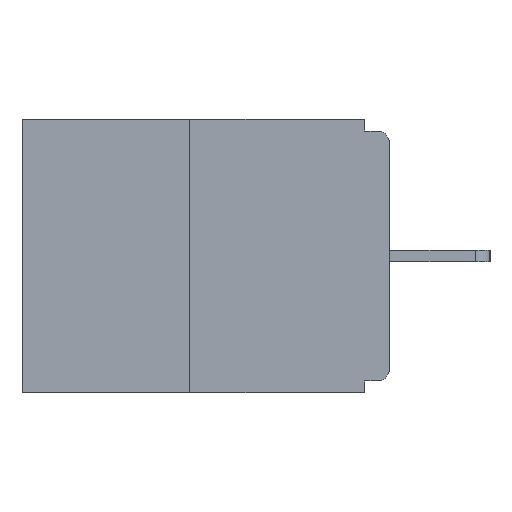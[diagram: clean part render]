
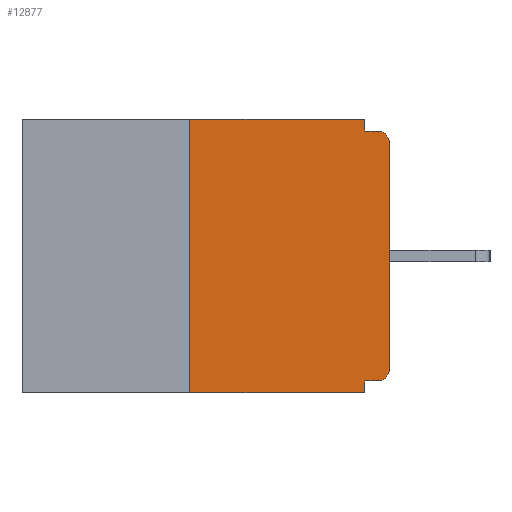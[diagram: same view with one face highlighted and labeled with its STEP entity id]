
A CAD part, left-side view. The second image highlights one B-rep face of the part: STEP entity #12877.
In plain terms, the highlighted planar face has unit normal (-1, 0, 0).
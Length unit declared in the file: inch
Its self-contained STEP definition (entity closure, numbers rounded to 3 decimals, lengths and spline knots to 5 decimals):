
#268 = EDGE_CURVE ( 'NONE', #17005, #15271, #13003, .T. ) ;
#376 = EDGE_CURVE ( 'NONE', #23818, #16217, #7460, .T. ) ;
#537 = LINE ( 'NONE', #25240, #22893 ) ;
#1853 = DIRECTION ( 'NONE',  ( 0., 0., 1. ) ) ;
#2669 = VECTOR ( 'NONE', #3980, 39.37008 ) ;
#2848 = DIRECTION ( 'NONE',  ( 0., 0., -1. ) ) ;
#2906 = VERTEX_POINT ( 'NONE', #8200 ) ;
#3591 = CIRCLE ( 'NONE', #9228, 0.015 ) ;
#3841 = CARTESIAN_POINT ( 'NONE',  ( 0., 0.015, -0.328 ) ) ;
#3980 = DIRECTION ( 'NONE',  ( 0., 0., -1. ) ) ;
#4024 = CARTESIAN_POINT ( 'NONE',  ( 0., 0., 0. ) ) ;
#4127 = AXIS2_PLACEMENT_3D ( 'NONE', #17732, #13574, #5185 ) ;
#4863 = CARTESIAN_POINT ( 'NONE',  ( 0., 0.015, -0.015 ) ) ;
#5080 = FACE_OUTER_BOUND ( 'NONE', #23691, .T. ) ;
#5173 = VECTOR ( 'NONE', #19610, 39.37008 ) ;
#5185 = DIRECTION ( 'NONE',  ( 0., 0., -1. ) ) ;
#5927 = VECTOR ( 'NONE', #1853, 39.37008 ) ;
#6051 = ORIENTED_EDGE ( 'NONE', *, *, #376, .F. ) ;
#6130 = EDGE_CURVE ( 'NONE', #23818, #2906, #10619, .T. ) ;
#6712 = VECTOR ( 'NONE', #8015, 39.37008 ) ;
#7460 = LINE ( 'NONE', #13792, #6712 ) ;
#8015 = DIRECTION ( 'NONE',  ( 0., 1., 0. ) ) ;
#8200 = CARTESIAN_POINT ( 'NONE',  ( 0., 0., -0.313 ) ) ;
#9228 = AXIS2_PLACEMENT_3D ( 'NONE', #24855, #12466, #20682 ) ;
#9291 = EDGE_CURVE ( 'NONE', #2906, #23727, #24266, .T. ) ;
#9389 = CARTESIAN_POINT ( 'NONE',  ( 0., 0.25, 0. ) ) ;
#9894 = CARTESIAN_POINT ( 'NONE',  ( 0., 0.031, 0. ) ) ;
#9942 = ORIENTED_EDGE ( 'NONE', *, *, #14783, .F. ) ;
#10184 = VECTOR ( 'NONE', #25661, 39.37008 ) ;
#10459 = DIRECTION ( 'NONE',  ( 0., -1., 0. ) ) ;
#10619 = CIRCLE ( 'NONE', #4127, 0.015 ) ;
#11185 = DIRECTION ( 'NONE',  ( 0., 0., -1. ) ) ;
#11404 = LINE ( 'NONE', #9389, #5173 ) ;
#11454 = DIRECTION ( 'NONE',  ( 1., 0., 0. ) ) ;
#11769 = VERTEX_POINT ( 'NONE', #14636 ) ;
#12466 = DIRECTION ( 'NONE',  ( -1., 0., 0. ) ) ;
#12542 = ORIENTED_EDGE ( 'NONE', *, *, #268, .F. ) ;
#12877 = ADVANCED_FACE ( 'NONE', ( #5080 ), #23568, .F. ) ;
#12882 = CARTESIAN_POINT ( 'NONE',  ( 0., 0.031, -0.328 ) ) ;
#13003 = LINE ( 'NONE', #17577, #10184 ) ;
#13457 = CARTESIAN_POINT ( 'NONE',  ( 0., 0.46, 0. ) ) ;
#13574 = DIRECTION ( 'NONE',  ( -1., 0., 0. ) ) ;
#13792 = CARTESIAN_POINT ( 'NONE',  ( 0., 0., -0.328 ) ) ;
#14130 = EDGE_CURVE ( 'NONE', #24259, #18812, #537, .T. ) ;
#14636 = CARTESIAN_POINT ( 'NONE',  ( 0., 0.031, -0.343 ) ) ;
#14783 = EDGE_CURVE ( 'NONE', #18812, #17005, #16258, .T. ) ;
#15094 = ORIENTED_EDGE ( 'NONE', *, *, #17762, .T. ) ;
#15271 = VERTEX_POINT ( 'NONE', #4863 ) ;
#15834 = ORIENTED_EDGE ( 'NONE', *, *, #25152, .T. ) ;
#16217 = VERTEX_POINT ( 'NONE', #12882 ) ;
#16241 = EDGE_CURVE ( 'NONE', #16217, #11769, #25123, .T. ) ;
#16258 = LINE ( 'NONE', #24494, #2669 ) ;
#16905 = CARTESIAN_POINT ( 'NONE',  ( 0., 0.25, -0.343 ) ) ;
#17005 = VERTEX_POINT ( 'NONE', #21390 ) ;
#17158 = CARTESIAN_POINT ( 'NONE',  ( 0., 0.031, -0.343 ) ) ;
#17433 = ORIENTED_EDGE ( 'NONE', *, *, #9291, .T. ) ;
#17577 = CARTESIAN_POINT ( 'NONE',  ( 0., 0., -0.015 ) ) ;
#17586 = ORIENTED_EDGE ( 'NONE', *, *, #6130, .T. ) ;
#17732 = CARTESIAN_POINT ( 'NONE',  ( 0., 0.015, -0.313 ) ) ;
#17762 = EDGE_CURVE ( 'NONE', #23727, #15271, #3591, .T. ) ;
#18196 = VERTEX_POINT ( 'NONE', #16905 ) ;
#18395 = EDGE_CURVE ( 'NONE', #18196, #24259, #11404, .T. ) ;
#18812 = VERTEX_POINT ( 'NONE', #9894 ) ;
#19480 = VECTOR ( 'NONE', #2848, 39.37008 ) ;
#19610 = DIRECTION ( 'NONE',  ( 0., 0., 1. ) ) ;
#20682 = DIRECTION ( 'NONE',  ( 0., 0., -1. ) ) ;
#21390 = CARTESIAN_POINT ( 'NONE',  ( 0., 0.031, -0.015 ) ) ;
#21612 = ORIENTED_EDGE ( 'NONE', *, *, #18395, .F. ) ;
#22893 = VECTOR ( 'NONE', #10459, 39.37008 ) ;
#23568 = PLANE ( 'NONE',  #24599 ) ;
#23691 = EDGE_LOOP ( 'NONE', ( #23769, #21612, #15834, #26125, #6051, #17586, #17433, #15094, #12542, #9942 ) ) ;
#23727 = VERTEX_POINT ( 'NONE', #25358 ) ;
#23769 = ORIENTED_EDGE ( 'NONE', *, *, #14130, .F. ) ;
#23818 = VERTEX_POINT ( 'NONE', #3841 ) ;
#23917 = CARTESIAN_POINT ( 'NONE',  ( 0., 0.25, 0. ) ) ;
#23953 = CARTESIAN_POINT ( 'NONE',  ( 0., 0.46, -0.343 ) ) ;
#24213 = LINE ( 'NONE', #23953, #25559 ) ;
#24259 = VERTEX_POINT ( 'NONE', #23917 ) ;
#24266 = LINE ( 'NONE', #4024, #5927 ) ;
#24494 = CARTESIAN_POINT ( 'NONE',  ( 0., 0.031, 0. ) ) ;
#24599 = AXIS2_PLACEMENT_3D ( 'NONE', #13457, #11454, #11185 ) ;
#24855 = CARTESIAN_POINT ( 'NONE',  ( 0., 0.015, -0.03 ) ) ;
#25123 = LINE ( 'NONE', #17158, #19480 ) ;
#25152 = EDGE_CURVE ( 'NONE', #18196, #11769, #24213, .T. ) ;
#25240 = CARTESIAN_POINT ( 'NONE',  ( 0., 0.46, 0. ) ) ;
#25358 = CARTESIAN_POINT ( 'NONE',  ( 0., 0., -0.03 ) ) ;
#25559 = VECTOR ( 'NONE', #26112, 39.37008 ) ;
#25661 = DIRECTION ( 'NONE',  ( 0., -1., 0. ) ) ;
#26112 = DIRECTION ( 'NONE',  ( 0., -1., 0. ) ) ;
#26125 = ORIENTED_EDGE ( 'NONE', *, *, #16241, .F. ) ;
